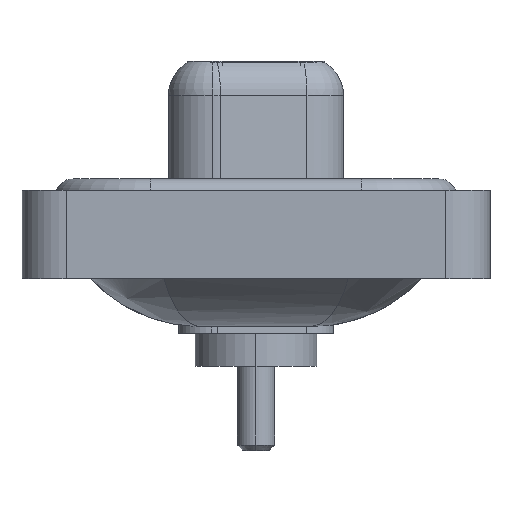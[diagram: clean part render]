
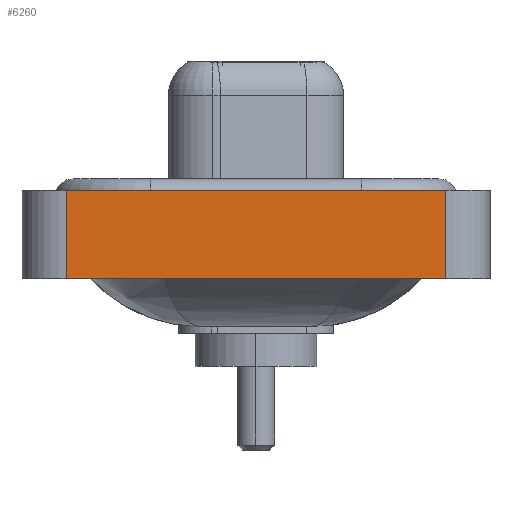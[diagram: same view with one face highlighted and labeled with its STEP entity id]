
A CAD part, left-side view. The second image highlights one B-rep face of the part: STEP entity #6260.
In plain terms, the highlighted planar face has unit normal (-1, 0, 0).
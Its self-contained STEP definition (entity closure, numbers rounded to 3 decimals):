
#866 = LINE ( 'NONE', #11695, #8251 ) ;
#3180 = CARTESIAN_POINT ( 'NONE',  ( -7.3, 8.55, 0.4 ) ) ;
#3397 = CARTESIAN_POINT ( 'NONE',  ( -7.3, 8.55, -3.6 ) ) ;
#3694 = VECTOR ( 'NONE', #10756, 1000. ) ;
#3835 = CARTESIAN_POINT ( 'NONE',  ( -7.3, -8.55, -3.6 ) ) ;
#4306 = AXIS2_PLACEMENT_3D ( 'NONE', #15349, #16799, #9000 ) ;
#4433 = EDGE_CURVE ( 'NONE', #8802, #6913, #16055, .T. ) ;
#4473 = ORIENTED_EDGE ( 'NONE', *, *, #7940, .T. ) ;
#5849 = FACE_OUTER_BOUND ( 'NONE', #13343, .T. ) ;
#6260 = ADVANCED_FACE ( 'NONE', ( #5849 ), #11285, .T. ) ;
#6359 = DIRECTION ( 'NONE',  ( 0., -1., 0. ) ) ;
#6521 = ORIENTED_EDGE ( 'NONE', *, *, #7398, .F. ) ;
#6913 = VERTEX_POINT ( 'NONE', #8658 ) ;
#7398 = EDGE_CURVE ( 'NONE', #12605, #8802, #866, .T. ) ;
#7687 = CARTESIAN_POINT ( 'NONE',  ( -7.3, -8.55, -3.6 ) ) ;
#7750 = DIRECTION ( 'NONE',  ( 0., 0., 1. ) ) ;
#7753 = LINE ( 'NONE', #3835, #8253 ) ;
#7940 = EDGE_CURVE ( 'NONE', #12605, #9562, #7753, .T. ) ;
#7976 = CARTESIAN_POINT ( 'NONE',  ( -7.3, -8.55, 0.4 ) ) ;
#8251 = VECTOR ( 'NONE', #7750, 1000. ) ;
#8253 = VECTOR ( 'NONE', #6359, 1000. ) ;
#8658 = CARTESIAN_POINT ( 'NONE',  ( -7.3, -8.55, 0.4 ) ) ;
#8802 = VERTEX_POINT ( 'NONE', #3180 ) ;
#9000 = DIRECTION ( 'NONE',  ( 0., 0., 1. ) ) ;
#9562 = VERTEX_POINT ( 'NONE', #16504 ) ;
#10019 = ORIENTED_EDGE ( 'NONE', *, *, #4433, .F. ) ;
#10756 = DIRECTION ( 'NONE',  ( 0., 0., 1. ) ) ;
#10798 = ORIENTED_EDGE ( 'NONE', *, *, #14236, .T. ) ;
#10950 = DIRECTION ( 'NONE',  ( 0., -1., 0. ) ) ;
#11285 = PLANE ( 'NONE',  #4306 ) ;
#11695 = CARTESIAN_POINT ( 'NONE',  ( -7.3, 8.55, -3.6 ) ) ;
#12605 = VERTEX_POINT ( 'NONE', #3397 ) ;
#13343 = EDGE_LOOP ( 'NONE', ( #10798, #10019, #6521, #4473 ) ) ;
#14236 = EDGE_CURVE ( 'NONE', #9562, #6913, #14507, .T. ) ;
#14507 = LINE ( 'NONE', #7687, #3694 ) ;
#15349 = CARTESIAN_POINT ( 'NONE',  ( -7.3, -8.55, -3.6 ) ) ;
#16055 = LINE ( 'NONE', #7976, #16456 ) ;
#16456 = VECTOR ( 'NONE', #10950, 1000. ) ;
#16504 = CARTESIAN_POINT ( 'NONE',  ( -7.3, -8.55, -3.6 ) ) ;
#16799 = DIRECTION ( 'NONE',  ( -1., 0., 0. ) ) ;
